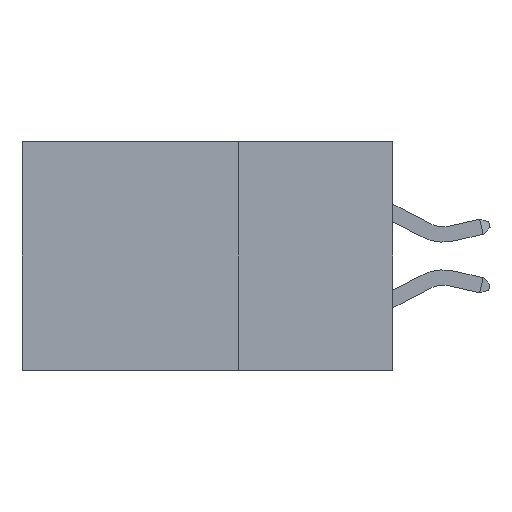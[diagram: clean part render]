
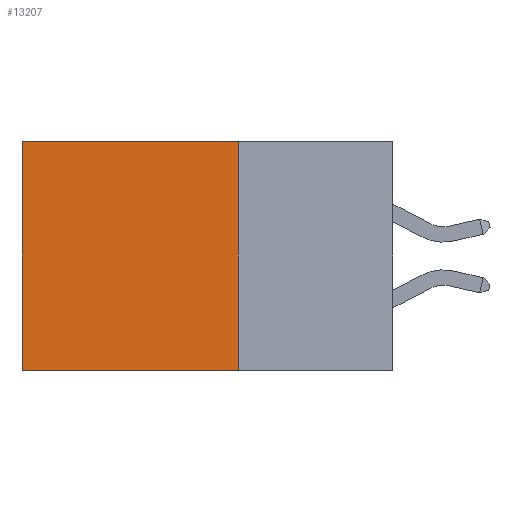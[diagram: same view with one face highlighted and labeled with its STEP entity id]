
A CAD part, left-side view. The second image highlights one B-rep face of the part: STEP entity #13207.
In plain terms, the highlighted planar face has unit normal (-1, 0, 0).
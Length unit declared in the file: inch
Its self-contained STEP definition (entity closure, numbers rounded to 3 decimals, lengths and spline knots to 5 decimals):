
#720 = VECTOR ( 'NONE', #8127, 39.37008 ) ;
#860 = DIRECTION ( 'NONE',  ( 1., 0., 0. ) ) ;
#2724 = VECTOR ( 'NONE', #12881, 39.37008 ) ;
#2839 = CARTESIAN_POINT ( 'NONE',  ( 0.2875, 0.25, 0. ) ) ;
#2894 = DIRECTION ( 'NONE',  ( 0., 0., -1. ) ) ;
#3123 = LINE ( 'NONE', #2839, #2724 ) ;
#3661 = LINE ( 'NONE', #15571, #720 ) ;
#3812 = CARTESIAN_POINT ( 'NONE',  ( 0.2875, 0.6, -0.37 ) ) ;
#4579 = EDGE_CURVE ( 'NONE', #4742, #4829, #3123, .T. ) ;
#4742 = VERTEX_POINT ( 'NONE', #9434 ) ;
#4829 = VERTEX_POINT ( 'NONE', #15768 ) ;
#5022 = VECTOR ( 'NONE', #2894, 39.37008 ) ;
#5462 = ORIENTED_EDGE ( 'NONE', *, *, #15290, .T. ) ;
#5956 = VECTOR ( 'NONE', #6613, 39.37008 ) ;
#6044 = EDGE_CURVE ( 'NONE', #4742, #15795, #3661, .T. ) ;
#6426 = CARTESIAN_POINT ( 'NONE',  ( 0.2875, 0.25, -0.37 ) ) ;
#6613 = DIRECTION ( 'NONE',  ( 0., 1., 0. ) ) ;
#7150 = CARTESIAN_POINT ( 'NONE',  ( 0.2875, 0.25, 0. ) ) ;
#7906 = CARTESIAN_POINT ( 'NONE',  ( 0.2875, 0.6, 0. ) ) ;
#8015 = FACE_OUTER_BOUND ( 'NONE', #11597, .T. ) ;
#8127 = DIRECTION ( 'NONE',  ( 0., 0., -1. ) ) ;
#8900 = EDGE_CURVE ( 'NONE', #15795, #13951, #12657, .T. ) ;
#9434 = CARTESIAN_POINT ( 'NONE',  ( 0.2875, 0.25, 0. ) ) ;
#9659 = DIRECTION ( 'NONE',  ( 0., 0., -1. ) ) ;
#10708 = AXIS2_PLACEMENT_3D ( 'NONE', #7150, #860, #9659 ) ;
#11012 = ORIENTED_EDGE ( 'NONE', *, *, #6044, .F. ) ;
#11567 = CARTESIAN_POINT ( 'NONE',  ( 0.2875, 0.25, -0.37 ) ) ;
#11597 = EDGE_LOOP ( 'NONE', ( #5462, #11929, #11012, #13365 ) ) ;
#11717 = LINE ( 'NONE', #7906, #5022 ) ;
#11929 = ORIENTED_EDGE ( 'NONE', *, *, #8900, .F. ) ;
#12657 = LINE ( 'NONE', #11567, #5956 ) ;
#12881 = DIRECTION ( 'NONE',  ( 0., 1., 0. ) ) ;
#13207 = ADVANCED_FACE ( 'NONE', ( #8015 ), #15820, .F. ) ;
#13365 = ORIENTED_EDGE ( 'NONE', *, *, #4579, .T. ) ;
#13951 = VERTEX_POINT ( 'NONE', #3812 ) ;
#15290 = EDGE_CURVE ( 'NONE', #4829, #13951, #11717, .T. ) ;
#15571 = CARTESIAN_POINT ( 'NONE',  ( 0.2875, 0.25, 0. ) ) ;
#15768 = CARTESIAN_POINT ( 'NONE',  ( 0.2875, 0.6, 0. ) ) ;
#15795 = VERTEX_POINT ( 'NONE', #6426 ) ;
#15820 = PLANE ( 'NONE',  #10708 ) ;
